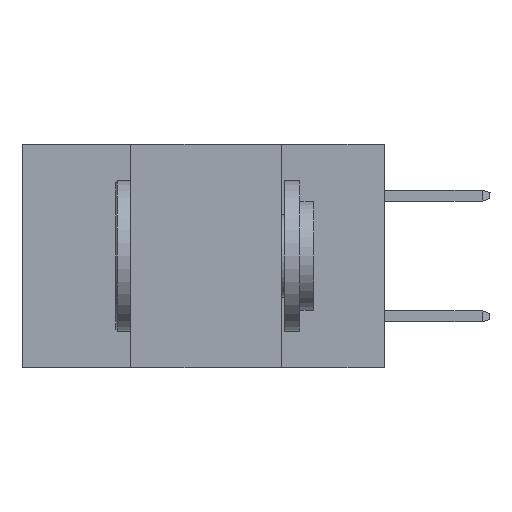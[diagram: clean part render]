
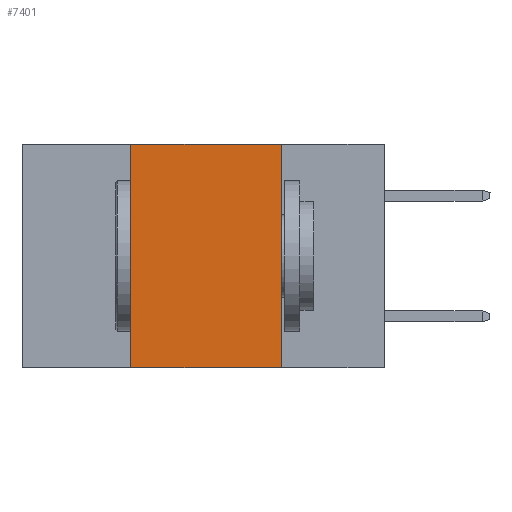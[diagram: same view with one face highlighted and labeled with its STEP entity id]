
A CAD part, left-side view. The second image highlights one B-rep face of the part: STEP entity #7401.
In plain terms, the highlighted planar face has unit normal (-1, 0, 0).
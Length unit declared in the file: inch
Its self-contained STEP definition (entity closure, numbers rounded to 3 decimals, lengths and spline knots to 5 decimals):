
#5 = CARTESIAN_POINT ( 'NONE',  ( 0., 0.42, -0.37 ) ) ;
#239 = VECTOR ( 'NONE', #10578, 39.37008 ) ;
#734 = AXIS2_PLACEMENT_3D ( 'NONE', #3180, #5848, #4079 ) ;
#970 = ORIENTED_EDGE ( 'NONE', *, *, #6112, .T. ) ;
#1537 = VECTOR ( 'NONE', #8605, 39.37008 ) ;
#1765 = CARTESIAN_POINT ( 'NONE',  ( 0., 0.17, 0. ) ) ;
#1792 = CARTESIAN_POINT ( 'NONE',  ( 0., 0.6, -0.37 ) ) ;
#1906 = VECTOR ( 'NONE', #2686, 39.37008 ) ;
#2443 = DIRECTION ( 'NONE',  ( 0., 0., 1. ) ) ;
#2495 = VECTOR ( 'NONE', #2443, 39.37008 ) ;
#2686 = DIRECTION ( 'NONE',  ( 0., -1., 0. ) ) ;
#2753 = CARTESIAN_POINT ( 'NONE',  ( 0., 0.17, -0.37 ) ) ;
#2950 = ORIENTED_EDGE ( 'NONE', *, *, #4175, .F. ) ;
#3180 = CARTESIAN_POINT ( 'NONE',  ( 0., 0.6, 0. ) ) ;
#3523 = VERTEX_POINT ( 'NONE', #5593 ) ;
#4063 = ORIENTED_EDGE ( 'NONE', *, *, #4842, .F. ) ;
#4079 = DIRECTION ( 'NONE',  ( 0., 0., -1. ) ) ;
#4175 = EDGE_CURVE ( 'NONE', #8445, #10453, #7221, .T. ) ;
#4842 = EDGE_CURVE ( 'NONE', #10453, #3523, #5545, .T. ) ;
#5545 = LINE ( 'NONE', #7658, #1537 ) ;
#5584 = LINE ( 'NONE', #1765, #239 ) ;
#5593 = CARTESIAN_POINT ( 'NONE',  ( 0., 0.17, 0. ) ) ;
#5848 = DIRECTION ( 'NONE',  ( 1., 0., 0. ) ) ;
#5920 = CARTESIAN_POINT ( 'NONE',  ( 0., 0.42, 0. ) ) ;
#5932 = PLANE ( 'NONE',  #734 ) ;
#6112 = EDGE_CURVE ( 'NONE', #8445, #7503, #7596, .T. ) ;
#7221 = LINE ( 'NONE', #5920, #2495 ) ;
#7401 = ADVANCED_FACE ( 'NONE', ( #10802 ), #5932, .F. ) ;
#7482 = EDGE_LOOP ( 'NONE', ( #10210, #4063, #2950, #970 ) ) ;
#7503 = VERTEX_POINT ( 'NONE', #2753 ) ;
#7596 = LINE ( 'NONE', #1792, #1906 ) ;
#7658 = CARTESIAN_POINT ( 'NONE',  ( 0., 0.6, 0. ) ) ;
#8357 = CARTESIAN_POINT ( 'NONE',  ( 0., 0.42, 0. ) ) ;
#8445 = VERTEX_POINT ( 'NONE', #5 ) ;
#8605 = DIRECTION ( 'NONE',  ( 0., -1., 0. ) ) ;
#9411 = EDGE_CURVE ( 'NONE', #3523, #7503, #5584, .T. ) ;
#10210 = ORIENTED_EDGE ( 'NONE', *, *, #9411, .F. ) ;
#10453 = VERTEX_POINT ( 'NONE', #8357 ) ;
#10578 = DIRECTION ( 'NONE',  ( 0., 0., -1. ) ) ;
#10802 = FACE_OUTER_BOUND ( 'NONE', #7482, .T. ) ;
